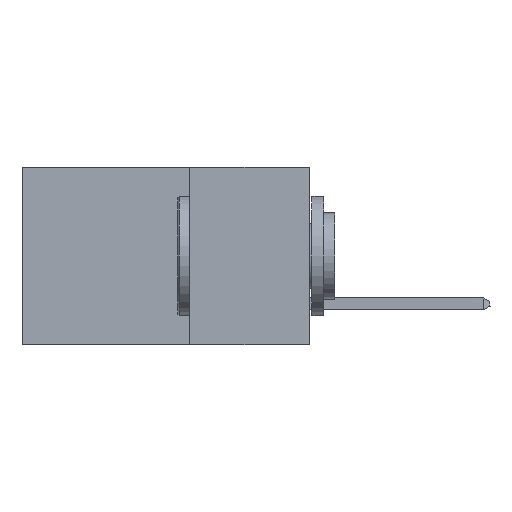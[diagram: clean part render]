
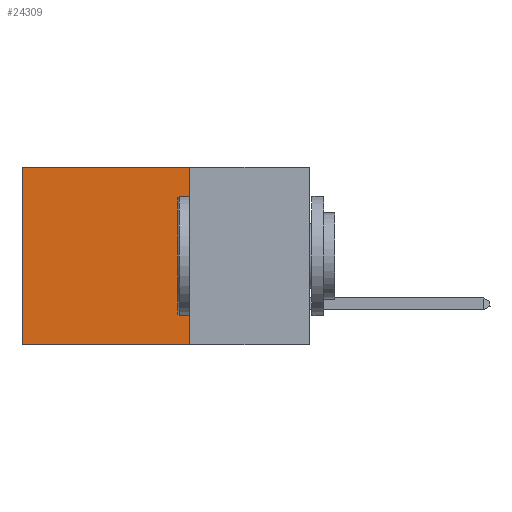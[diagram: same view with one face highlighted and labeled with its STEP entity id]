
A CAD part, left-side view. The second image highlights one B-rep face of the part: STEP entity #24309.
In plain terms, the highlighted planar face has unit normal (-1, 0, 0).
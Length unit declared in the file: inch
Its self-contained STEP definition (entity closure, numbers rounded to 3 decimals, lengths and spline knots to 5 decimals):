
#1116 = FACE_OUTER_BOUND ( 'NONE', #24038, .T. ) ;
#1660 = LINE ( 'NONE', #15355, #7978 ) ;
#1824 = LINE ( 'NONE', #11979, #6580 ) ;
#3121 = CARTESIAN_POINT ( 'NONE',  ( 0.2875, 0.6, 0. ) ) ;
#3672 = LINE ( 'NONE', #27606, #24347 ) ;
#4937 = DIRECTION ( 'NONE',  ( 0., 1., 0. ) ) ;
#5289 = ORIENTED_EDGE ( 'NONE', *, *, #18848, .F. ) ;
#6580 = VECTOR ( 'NONE', #24978, 39.37008 ) ;
#7978 = VECTOR ( 'NONE', #23047, 39.37008 ) ;
#8511 = ORIENTED_EDGE ( 'NONE', *, *, #12166, .T. ) ;
#9358 = EDGE_CURVE ( 'NONE', #15465, #10660, #1824, .T. ) ;
#10660 = VERTEX_POINT ( 'NONE', #15235 ) ;
#11335 = VERTEX_POINT ( 'NONE', #20812 ) ;
#11793 = LINE ( 'NONE', #15458, #30496 ) ;
#11979 = CARTESIAN_POINT ( 'NONE',  ( 0.2875, 0.6, 0. ) ) ;
#12166 = EDGE_CURVE ( 'NONE', #15837, #15465, #1660, .T. ) ;
#15142 = DIRECTION ( 'NONE',  ( 0., 0., -1. ) ) ;
#15235 = CARTESIAN_POINT ( 'NONE',  ( 0.2875, 0.6, -0.37 ) ) ;
#15355 = CARTESIAN_POINT ( 'NONE',  ( 0.2875, 0.25, 0. ) ) ;
#15458 = CARTESIAN_POINT ( 'NONE',  ( 0.2875, 0.25, -0.37 ) ) ;
#15465 = VERTEX_POINT ( 'NONE', #3121 ) ;
#15837 = VERTEX_POINT ( 'NONE', #23698 ) ;
#18848 = EDGE_CURVE ( 'NONE', #11335, #10660, #11793, .T. ) ;
#20812 = CARTESIAN_POINT ( 'NONE',  ( 0.2875, 0.25, -0.37 ) ) ;
#21117 = AXIS2_PLACEMENT_3D ( 'NONE', #25363, #27928, #15142 ) ;
#22931 = PLANE ( 'NONE',  #21117 ) ;
#23047 = DIRECTION ( 'NONE',  ( 0., 1., 0. ) ) ;
#23698 = CARTESIAN_POINT ( 'NONE',  ( 0.2875, 0.25, 0. ) ) ;
#24038 = EDGE_LOOP ( 'NONE', ( #25785, #5289, #32159, #8511 ) ) ;
#24309 = ADVANCED_FACE ( 'NONE', ( #1116 ), #22931, .F. ) ;
#24347 = VECTOR ( 'NONE', #30167, 39.37008 ) ;
#24978 = DIRECTION ( 'NONE',  ( 0., 0., -1. ) ) ;
#25363 = CARTESIAN_POINT ( 'NONE',  ( 0.2875, 0.25, 0. ) ) ;
#25682 = EDGE_CURVE ( 'NONE', #15837, #11335, #3672, .T. ) ;
#25785 = ORIENTED_EDGE ( 'NONE', *, *, #9358, .T. ) ;
#27606 = CARTESIAN_POINT ( 'NONE',  ( 0.2875, 0.25, 0. ) ) ;
#27928 = DIRECTION ( 'NONE',  ( 1., 0., 0. ) ) ;
#30167 = DIRECTION ( 'NONE',  ( 0., 0., -1. ) ) ;
#30496 = VECTOR ( 'NONE', #4937, 39.37008 ) ;
#32159 = ORIENTED_EDGE ( 'NONE', *, *, #25682, .F. ) ;
